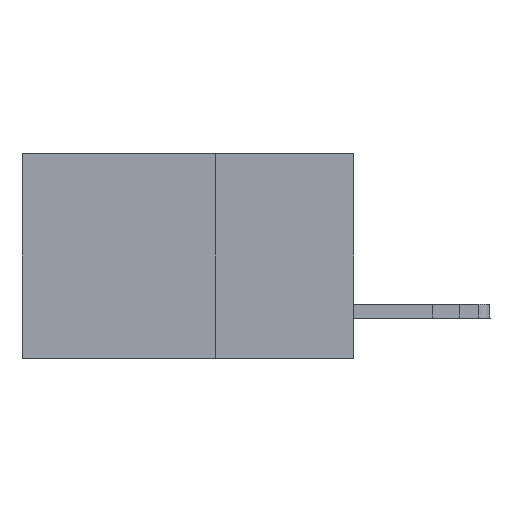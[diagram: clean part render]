
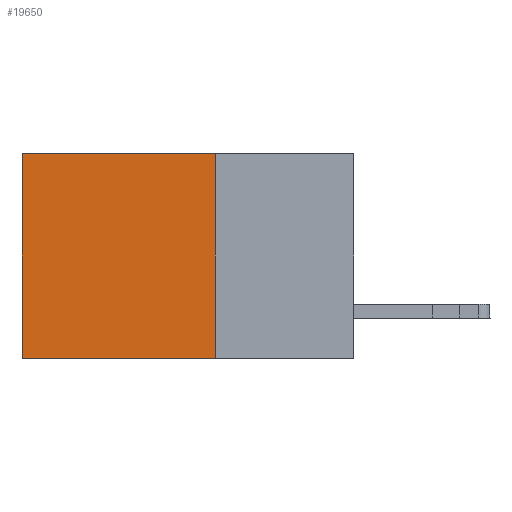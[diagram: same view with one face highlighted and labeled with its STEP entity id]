
A CAD part, left-side view. The second image highlights one B-rep face of the part: STEP entity #19650.
In plain terms, the highlighted planar face has unit normal (-1, 0, 0).
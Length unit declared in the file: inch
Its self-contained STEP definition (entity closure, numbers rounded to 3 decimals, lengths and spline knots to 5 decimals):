
#153 = CARTESIAN_POINT ( 'NONE',  ( 0.2875, 0.25, -0.37 ) ) ;
#519 = DIRECTION ( 'NONE',  ( 0., 1., 0. ) ) ;
#1524 = VERTEX_POINT ( 'NONE', #9603 ) ;
#2008 = DIRECTION ( 'NONE',  ( 1., 0., 0. ) ) ;
#2619 = VERTEX_POINT ( 'NONE', #8720 ) ;
#3057 = EDGE_CURVE ( 'NONE', #18196, #8918, #21023, .T. ) ;
#4031 = EDGE_CURVE ( 'NONE', #1524, #2619, #7095, .T. ) ;
#5327 = DIRECTION ( 'NONE',  ( 0., 0., -1. ) ) ;
#5546 = DIRECTION ( 'NONE',  ( 0., 0., -1. ) ) ;
#6093 = EDGE_CURVE ( 'NONE', #2619, #8918, #10589, .T. ) ;
#6161 = CARTESIAN_POINT ( 'NONE',  ( 0.2875, 0.6, 0. ) ) ;
#6359 = VECTOR ( 'NONE', #519, 39.37008 ) ;
#6883 = CARTESIAN_POINT ( 'NONE',  ( 0.2875, 0.25, 0. ) ) ;
#7095 = LINE ( 'NONE', #6883, #18728 ) ;
#7180 = ORIENTED_EDGE ( 'NONE', *, *, #9205, .T. ) ;
#7196 = PLANE ( 'NONE',  #10982 ) ;
#7666 = LINE ( 'NONE', #20986, #6359 ) ;
#7975 = ORIENTED_EDGE ( 'NONE', *, *, #6093, .F. ) ;
#8720 = CARTESIAN_POINT ( 'NONE',  ( 0.2875, 0.25, -0.37 ) ) ;
#8918 = VERTEX_POINT ( 'NONE', #15641 ) ;
#9205 = EDGE_CURVE ( 'NONE', #1524, #18196, #7666, .T. ) ;
#9603 = CARTESIAN_POINT ( 'NONE',  ( 0.2875, 0.25, 0. ) ) ;
#10364 = CARTESIAN_POINT ( 'NONE',  ( 0.2875, 0.25, 0. ) ) ;
#10589 = LINE ( 'NONE', #153, #17055 ) ;
#10774 = DIRECTION ( 'NONE',  ( 0., 0., -1. ) ) ;
#10982 = AXIS2_PLACEMENT_3D ( 'NONE', #10364, #2008, #5546 ) ;
#14181 = VECTOR ( 'NONE', #10774, 39.37008 ) ;
#15256 = DIRECTION ( 'NONE',  ( 0., 1., 0. ) ) ;
#15641 = CARTESIAN_POINT ( 'NONE',  ( 0.2875, 0.6, -0.37 ) ) ;
#17055 = VECTOR ( 'NONE', #15256, 39.37008 ) ;
#18196 = VERTEX_POINT ( 'NONE', #20133 ) ;
#18434 = ORIENTED_EDGE ( 'NONE', *, *, #3057, .T. ) ;
#18728 = VECTOR ( 'NONE', #5327, 39.37008 ) ;
#19650 = ADVANCED_FACE ( 'NONE', ( #20399 ), #7196, .F. ) ;
#19710 = EDGE_LOOP ( 'NONE', ( #18434, #7975, #19792, #7180 ) ) ;
#19792 = ORIENTED_EDGE ( 'NONE', *, *, #4031, .F. ) ;
#20133 = CARTESIAN_POINT ( 'NONE',  ( 0.2875, 0.6, 0. ) ) ;
#20399 = FACE_OUTER_BOUND ( 'NONE', #19710, .T. ) ;
#20986 = CARTESIAN_POINT ( 'NONE',  ( 0.2875, 0.25, 0. ) ) ;
#21023 = LINE ( 'NONE', #6161, #14181 ) ;
